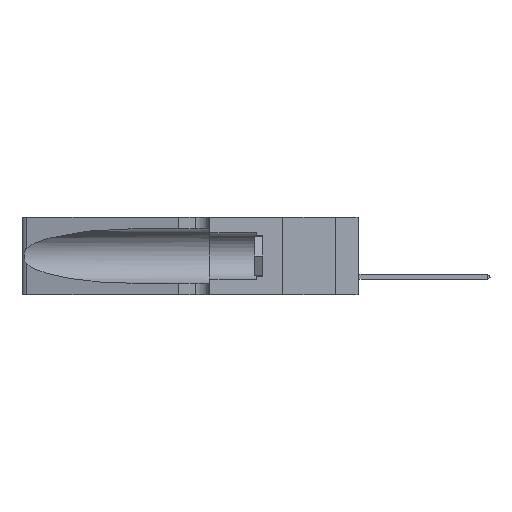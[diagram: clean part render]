
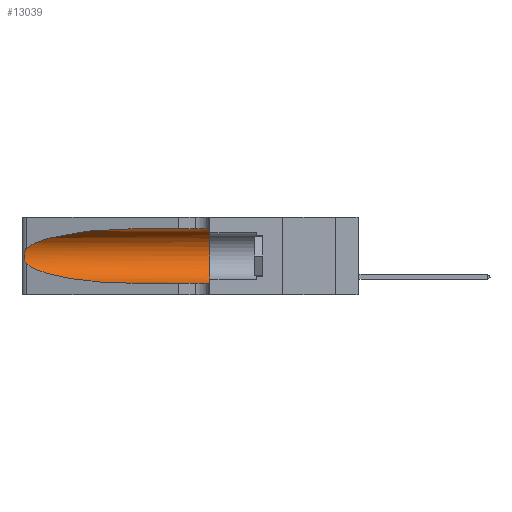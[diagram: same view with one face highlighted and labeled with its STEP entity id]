
A CAD part, left-side view. The second image highlights one B-rep face of the part: STEP entity #13039.
In plain terms, the highlighted cylindrical face has radius 3.308 mm (diameter 6.617 mm), a partial arc.
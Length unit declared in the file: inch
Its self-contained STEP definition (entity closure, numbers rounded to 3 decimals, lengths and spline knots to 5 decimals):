
#308 = AXIS2_PLACEMENT_3D ( 'NONE', #6942, #549, #20106 ) ;
#549 = DIRECTION ( 'NONE',  ( 0., 1., 0. ) ) ;
#772 = DIRECTION ( 'NONE',  ( 0., -1., 0. ) ) ;
#795 = CARTESIAN_POINT ( 'NONE',  ( 0.26017, 1.23833, 0.17102 ) ) ;
#1534 = EDGE_LOOP ( 'NONE', ( #24091, #1740, #7355, #16260, #4829, #1653 ) ) ;
#1653 = ORIENTED_EDGE ( 'NONE', *, *, #10049, .F. ) ;
#1740 = ORIENTED_EDGE ( 'NONE', *, *, #13150, .T. ) ;
#1948 = VECTOR ( 'NONE', #5026, 39.37008 ) ;
#1986 = CARTESIAN_POINT ( 'NONE',  ( 0.25487, 1.22718, 0.22369 ) ) ;
#2338 = AXIS2_PLACEMENT_3D ( 'NONE', #4743, #772, #18190 ) ;
#2621 = CARTESIAN_POINT ( 'NONE',  ( 0.26018, 1.23835, 0.19895 ) ) ;
#4001 = CARTESIAN_POINT ( 'NONE',  ( 0.1305, 0.35, 0.05475 ) ) ;
#4743 = CARTESIAN_POINT ( 'NONE',  ( 0.1305, 1.61858, 0.185 ) ) ;
#4829 = ORIENTED_EDGE ( 'NONE', *, *, #11837, .F. ) ;
#4990 = CARTESIAN_POINT ( 'NONE',  ( 0.1305, 0.72297, 0.05475 ) ) ;
#5026 = DIRECTION ( 'NONE',  ( 0., -1., 0. ) ) ;
#5075 = CARTESIAN_POINT ( 'NONE',  ( 0.25487, 1.22718, 0.14631 ) ) ;
#5494 = CYLINDRICAL_SURFACE ( 'NONE', #2338, 0.13025 ) ;
#5931 = EDGE_CURVE ( 'NONE', #11667, #9694, #11274, .T. ) ;
#6122 = EDGE_CURVE ( 'NONE', #16205, #17840, #20873, .T. ) ;
#6782 = CARTESIAN_POINT ( 'NONE',  ( 0.2373, 1.15595, 0.08982 ) ) ;
#6942 = CARTESIAN_POINT ( 'NONE',  ( 0.1305, 0.35, 0.185 ) ) ;
#7355 = ORIENTED_EDGE ( 'NONE', *, *, #21349, .T. ) ;
#8134 = VECTOR ( 'NONE', #20505, 39.37008 ) ;
#8363 = CARTESIAN_POINT ( 'NONE',  ( 0.25639, 1.23186, 0.15144 ) ) ;
#9694 = VERTEX_POINT ( 'NONE', #22681 ) ;
#9813 = CARTESIAN_POINT ( 'NONE',  ( 0.18966, 0.96281, 0.31525 ) ) ;
#10049 = EDGE_CURVE ( 'NONE', #11667, #22575, #22124, .T. ) ;
#10262 = CARTESIAN_POINT ( 'NONE',  ( 0.25787, 1.23484, 0.2124 ) ) ;
#10343 = CARTESIAN_POINT ( 'NONE',  ( 0.25487, 1.22718, 0.14631 ) ) ;
#10440 = CARTESIAN_POINT ( 'NONE',  ( 0.25487, 1.22718, 0.22369 ) ) ;
#10468 = CARTESIAN_POINT ( 'NONE',  ( 0.25487, 1.22718, 0.14631 ) ) ;
#11126 = CIRCLE ( 'NONE', #308, 0.13025 ) ;
#11274 =( BOUNDED_CURVE ( )  B_SPLINE_CURVE ( 3, ( #23456, #9813, #13723, #1986 ),
 .UNSPECIFIED., .F., .T. ) 
 B_SPLINE_CURVE_WITH_KNOTS ( ( 4, 4 ),
 ( 1.5708, 2.84003 ),
 .UNSPECIFIED. ) 
 CURVE ( )  GEOMETRIC_REPRESENTATION_ITEM ( )  RATIONAL_B_SPLINE_CURVE ( ( 1., 0.87, 0.87, 1. ) ) 
 REPRESENTATION_ITEM ( '' )  );
#11667 = VERTEX_POINT ( 'NONE', #22246 ) ;
#11837 = EDGE_CURVE ( 'NONE', #22575, #17840, #11126, .T. ) ;
#11900 = B_SPLINE_CURVE_WITH_KNOTS ( 'NONE', 3,
 ( #10440, #16115, #12559, #10262, #20258, #2621, #23903, #20170, #795, #14513, #23814, #8363, #21950, #10343 ),
 .UNSPECIFIED., .F., .F.,
 ( 4, 2, 2, 2, 2, 2, 4 ),
 ( 0., 0.00027, 0.00053, 0.00107, 0.0016, 0.00187, 0.00214 ),
 .UNSPECIFIED. ) ;
#12375 = CARTESIAN_POINT ( 'NONE',  ( 0.1305, 0.72297, 0.05475 ) ) ;
#12559 = CARTESIAN_POINT ( 'NONE',  ( 0.25639, 1.23184, 0.21858 ) ) ;
#13039 = ADVANCED_FACE ( 'NONE', ( #21382 ), #5494, .F. ) ;
#13150 = EDGE_CURVE ( 'NONE', #9694, #14865, #11900, .T. ) ;
#13723 = CARTESIAN_POINT ( 'NONE',  ( 0.2373, 1.15595, 0.28018 ) ) ;
#14448 = CARTESIAN_POINT ( 'NONE',  ( 0.1305, 1.61858, 0.05475 ) ) ;
#14513 = CARTESIAN_POINT ( 'NONE',  ( 0.25856, 1.23593, 0.16098 ) ) ;
#14865 = VERTEX_POINT ( 'NONE', #10468 ) ;
#14983 = CARTESIAN_POINT ( 'NONE',  ( 0.18966, 0.96281, 0.05475 ) ) ;
#16115 = CARTESIAN_POINT ( 'NONE',  ( 0.25555, 1.22994, 0.2215 ) ) ;
#16205 = VERTEX_POINT ( 'NONE', #12375 ) ;
#16260 = ORIENTED_EDGE ( 'NONE', *, *, #6122, .T. ) ;
#16787 = CARTESIAN_POINT ( 'NONE',  ( 0.1305, 1.61858, 0.31525 ) ) ;
#17840 = VERTEX_POINT ( 'NONE', #4001 ) ;
#18190 = DIRECTION ( 'NONE',  ( 0., 0., -1. ) ) ;
#20106 = DIRECTION ( 'NONE',  ( 0., 0., 1. ) ) ;
#20170 = CARTESIAN_POINT ( 'NONE',  ( 0.26075, 1.23896, 0.178 ) ) ;
#20258 = CARTESIAN_POINT ( 'NONE',  ( 0.25854, 1.2359, 0.20912 ) ) ;
#20505 = DIRECTION ( 'NONE',  ( 0., -1., 0. ) ) ;
#20873 = LINE ( 'NONE', #14448, #1948 ) ;
#21349 = EDGE_CURVE ( 'NONE', #14865, #16205, #21963, .T. ) ;
#21382 = FACE_OUTER_BOUND ( 'NONE', #1534, .T. ) ;
#21859 = CARTESIAN_POINT ( 'NONE',  ( 0.1305, 0.35, 0.31525 ) ) ;
#21950 = CARTESIAN_POINT ( 'NONE',  ( 0.25555, 1.22993, 0.14849 ) ) ;
#21963 =( BOUNDED_CURVE ( )  B_SPLINE_CURVE ( 3, ( #5075, #6782, #14983, #4990 ),
 .UNSPECIFIED., .F., .T. ) 
 B_SPLINE_CURVE_WITH_KNOTS ( ( 4, 4 ),
 ( 3.44316, 4.71239 ),
 .UNSPECIFIED. ) 
 CURVE ( )  GEOMETRIC_REPRESENTATION_ITEM ( )  RATIONAL_B_SPLINE_CURVE ( ( 1., 0.87, 0.87, 1. ) ) 
 REPRESENTATION_ITEM ( '' )  );
#22124 = LINE ( 'NONE', #16787, #8134 ) ;
#22246 = CARTESIAN_POINT ( 'NONE',  ( 0.1305, 0.72297, 0.31525 ) ) ;
#22575 = VERTEX_POINT ( 'NONE', #21859 ) ;
#22681 = CARTESIAN_POINT ( 'NONE',  ( 0.25487, 1.22718, 0.22369 ) ) ;
#23456 = CARTESIAN_POINT ( 'NONE',  ( 0.1305, 0.72297, 0.31525 ) ) ;
#23814 = CARTESIAN_POINT ( 'NONE',  ( 0.25789, 1.23486, 0.15765 ) ) ;
#23903 = CARTESIAN_POINT ( 'NONE',  ( 0.26075, 1.23896, 0.19203 ) ) ;
#24091 = ORIENTED_EDGE ( 'NONE', *, *, #5931, .T. ) ;
